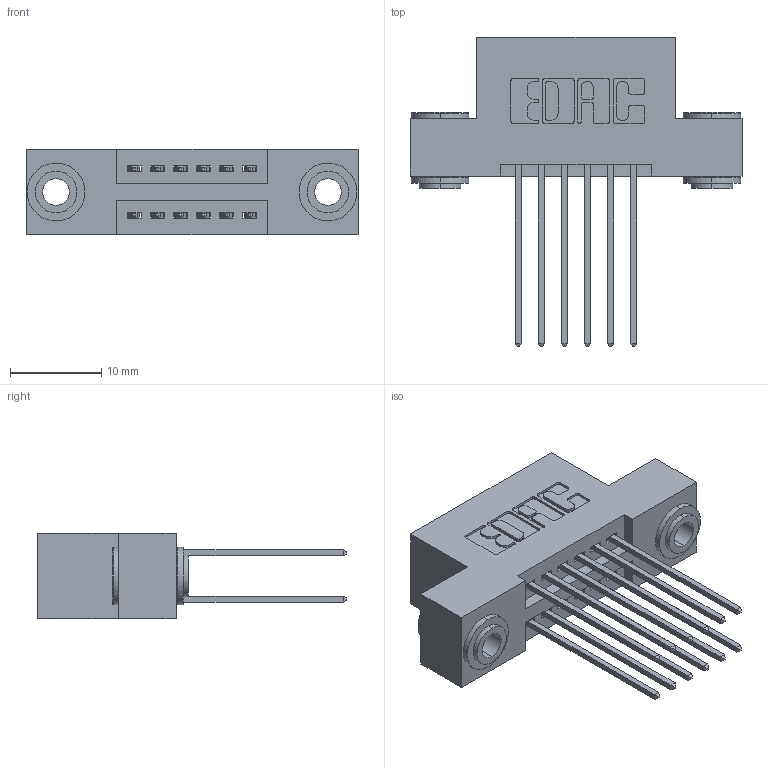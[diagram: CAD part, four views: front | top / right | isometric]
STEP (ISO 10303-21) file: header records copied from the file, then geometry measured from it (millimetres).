
FILE_DESCRIPTION (( 'STEP AP203' ), '1' );
FILE_NAME ('345-012-541-203.STEP', '2019-10-26T16:08:37', ( '' ), ( '' ), 'SwSTEP 2.0', 'SolidWorks 2016', '' );
FILE_SCHEMA (( 'CONFIG_CONTROL_DESIGN' ));
Length unit declared in the file: inch
Products named in the file (4): 345 Part_Flush Mounting Lugs - 0.156 Dia-TH; 345-012-541-203; 345-292-001_345-293-141; 345-250-002_345-250-002-102
Assembly tree (15 placements, depth 2):
  345-012-541-203
    345 Part_Flush Mounting Lugs - 0.156 Dia-TH
    345-292-001_345-293-141  x12
    345-250-002_345-250-002-102  x2
Bounding box: 36.45 x 33.96 x 9.4 mm (x, y, z)
Volume: 3294.8 mm3; surface area: 4701.5 mm2
Topology: 15 solids, 15 shells, 764 faces, 2205 edges, 1450 vertices
Faces by surface type: plane 486, cylinder 270, cone 8
Entity records: 10222 total; most frequent: CARTESIAN_POINT 1723, ORIENTED_EDGE 1650, DIRECTION 1595, EDGE_CURVE 825, LINE 645, VECTOR 645, VERTEX_POINT 546, AXIS2_PLACEMENT_3D 475
